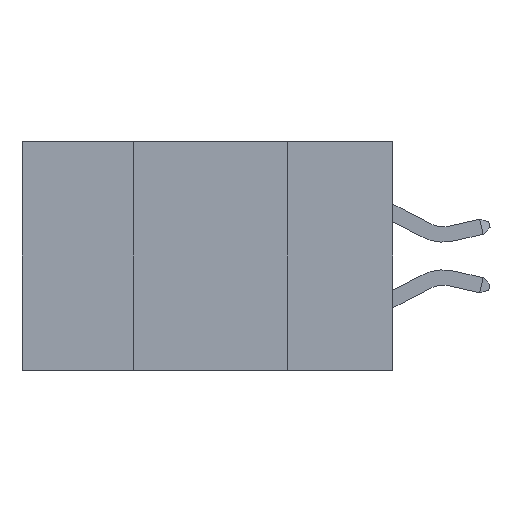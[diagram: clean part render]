
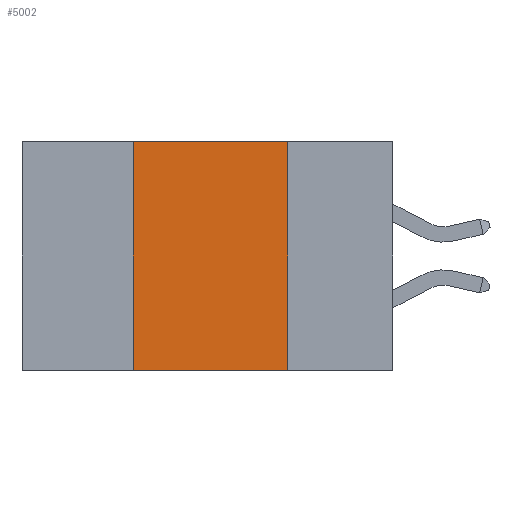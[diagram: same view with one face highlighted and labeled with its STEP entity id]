
A CAD part, left-side view. The second image highlights one B-rep face of the part: STEP entity #5002.
In plain terms, the highlighted planar face has unit normal (-1, 0, 0).
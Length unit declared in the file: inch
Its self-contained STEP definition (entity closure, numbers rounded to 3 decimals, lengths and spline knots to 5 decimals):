
#494 = EDGE_LOOP ( 'NONE', ( #5907, #7869, #7285, #15399 ) ) ;
#1550 = LINE ( 'NONE', #10538, #10260 ) ;
#2271 = EDGE_CURVE ( 'NONE', #4791, #20251, #7100, .T. ) ;
#2365 = CARTESIAN_POINT ( 'NONE',  ( 0., 0.6, -0.37 ) ) ;
#2466 = VECTOR ( 'NONE', #2908, 39.37008 ) ;
#2908 = DIRECTION ( 'NONE',  ( 0., -1., 0. ) ) ;
#3414 = DIRECTION ( 'NONE',  ( 1., 0., 0. ) ) ;
#3634 = DIRECTION ( 'NONE',  ( 0., 0., -1. ) ) ;
#4791 = VERTEX_POINT ( 'NONE', #12760 ) ;
#5002 = ADVANCED_FACE ( 'NONE', ( #6435 ), #9440, .F. ) ;
#5005 = CARTESIAN_POINT ( 'NONE',  ( 0., 0.42, 0. ) ) ;
#5907 = ORIENTED_EDGE ( 'NONE', *, *, #20642, .F. ) ;
#6036 = CARTESIAN_POINT ( 'NONE',  ( 0., 0.17, -0.37 ) ) ;
#6299 = CARTESIAN_POINT ( 'NONE',  ( 0., 0.42, 0. ) ) ;
#6435 = FACE_OUTER_BOUND ( 'NONE', #494, .T. ) ;
#6960 = DIRECTION ( 'NONE',  ( 0., -1., 0. ) ) ;
#7059 = DIRECTION ( 'NONE',  ( 0., 0., -1. ) ) ;
#7100 = LINE ( 'NONE', #2365, #2466 ) ;
#7285 = ORIENTED_EDGE ( 'NONE', *, *, #15034, .F. ) ;
#7869 = ORIENTED_EDGE ( 'NONE', *, *, #15286, .F. ) ;
#9094 = VECTOR ( 'NONE', #6960, 39.37008 ) ;
#9440 = PLANE ( 'NONE',  #20730 ) ;
#10260 = VECTOR ( 'NONE', #3634, 39.37008 ) ;
#10418 = VERTEX_POINT ( 'NONE', #12551 ) ;
#10430 = CARTESIAN_POINT ( 'NONE',  ( 0., 0.6, 0. ) ) ;
#10538 = CARTESIAN_POINT ( 'NONE',  ( 0., 0.17, 0. ) ) ;
#10991 = LINE ( 'NONE', #6299, #14491 ) ;
#12551 = CARTESIAN_POINT ( 'NONE',  ( 0., 0.17, 0. ) ) ;
#12760 = CARTESIAN_POINT ( 'NONE',  ( 0., 0.42, -0.37 ) ) ;
#13153 = LINE ( 'NONE', #17209, #9094 ) ;
#14491 = VECTOR ( 'NONE', #18264, 39.37008 ) ;
#15034 = EDGE_CURVE ( 'NONE', #4791, #21036, #10991, .T. ) ;
#15286 = EDGE_CURVE ( 'NONE', #21036, #10418, #13153, .T. ) ;
#15399 = ORIENTED_EDGE ( 'NONE', *, *, #2271, .T. ) ;
#17209 = CARTESIAN_POINT ( 'NONE',  ( 0., 0.6, 0. ) ) ;
#18264 = DIRECTION ( 'NONE',  ( 0., 0., 1. ) ) ;
#20251 = VERTEX_POINT ( 'NONE', #6036 ) ;
#20642 = EDGE_CURVE ( 'NONE', #10418, #20251, #1550, .T. ) ;
#20730 = AXIS2_PLACEMENT_3D ( 'NONE', #10430, #3414, #7059 ) ;
#21036 = VERTEX_POINT ( 'NONE', #5005 ) ;
